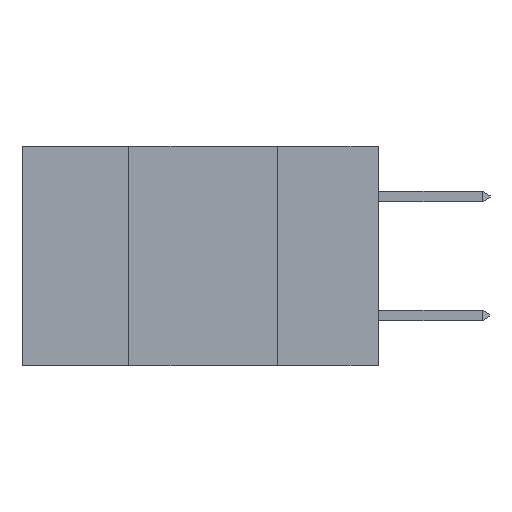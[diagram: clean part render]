
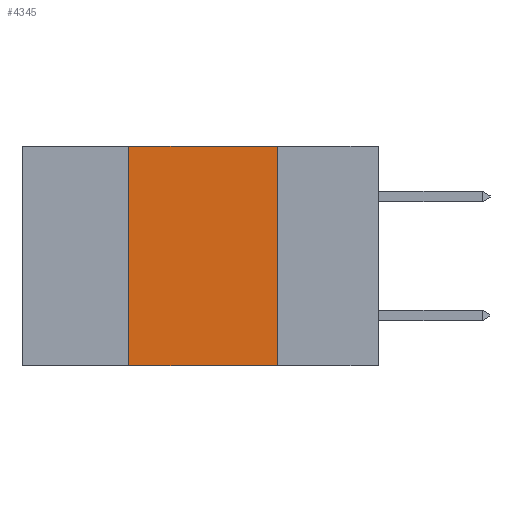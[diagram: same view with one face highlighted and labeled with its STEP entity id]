
A CAD part, left-side view. The second image highlights one B-rep face of the part: STEP entity #4345.
In plain terms, the highlighted planar face has unit normal (-1, 0, 0).
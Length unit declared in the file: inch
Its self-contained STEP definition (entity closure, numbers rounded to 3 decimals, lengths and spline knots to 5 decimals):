
#388 = LINE ( 'NONE', #13098, #13174 ) ;
#1026 = CARTESIAN_POINT ( 'NONE',  ( 0., 0.42, -0.37 ) ) ;
#1184 = VERTEX_POINT ( 'NONE', #21599 ) ;
#2242 = DIRECTION ( 'NONE',  ( 0., -1., 0. ) ) ;
#2478 = LINE ( 'NONE', #9098, #7949 ) ;
#3179 = FACE_OUTER_BOUND ( 'NONE', #18530, .T. ) ;
#3325 = ORIENTED_EDGE ( 'NONE', *, *, #21270, .T. ) ;
#3653 = DIRECTION ( 'NONE',  ( 0., -1., 0. ) ) ;
#3679 = CARTESIAN_POINT ( 'NONE',  ( 0., 0.17, 0. ) ) ;
#4157 = DIRECTION ( 'NONE',  ( 0., 0., -1. ) ) ;
#4345 = ADVANCED_FACE ( 'NONE', ( #3179 ), #14023, .F. ) ;
#6291 = VECTOR ( 'NONE', #14148, 39.37008 ) ;
#6836 = LINE ( 'NONE', #12364, #6291 ) ;
#7418 = VECTOR ( 'NONE', #2242, 39.37008 ) ;
#7736 = VERTEX_POINT ( 'NONE', #15699 ) ;
#7949 = VECTOR ( 'NONE', #3653, 39.37008 ) ;
#7960 = LINE ( 'NONE', #11292, #7418 ) ;
#9098 = CARTESIAN_POINT ( 'NONE',  ( 0., 0.6, 0. ) ) ;
#10260 = VERTEX_POINT ( 'NONE', #1026 ) ;
#11292 = CARTESIAN_POINT ( 'NONE',  ( 0., 0.6, -0.37 ) ) ;
#11504 = AXIS2_PLACEMENT_3D ( 'NONE', #13563, #13070, #12817 ) ;
#11874 = EDGE_CURVE ( 'NONE', #12886, #7736, #388, .T. ) ;
#12364 = CARTESIAN_POINT ( 'NONE',  ( 0., 0.42, -0.37 ) ) ;
#12817 = DIRECTION ( 'NONE',  ( 0., 0., -1. ) ) ;
#12886 = VERTEX_POINT ( 'NONE', #3679 ) ;
#13070 = DIRECTION ( 'NONE',  ( 1., 0., 0. ) ) ;
#13098 = CARTESIAN_POINT ( 'NONE',  ( 0., 0.17, -0.37 ) ) ;
#13174 = VECTOR ( 'NONE', #4157, 39.37008 ) ;
#13463 = ORIENTED_EDGE ( 'NONE', *, *, #18896, .F. ) ;
#13563 = CARTESIAN_POINT ( 'NONE',  ( 0., 0.6, 0. ) ) ;
#14023 = PLANE ( 'NONE',  #11504 ) ;
#14148 = DIRECTION ( 'NONE',  ( 0., 0., 1. ) ) ;
#14541 = ORIENTED_EDGE ( 'NONE', *, *, #11874, .F. ) ;
#15699 = CARTESIAN_POINT ( 'NONE',  ( 0., 0.17, -0.37 ) ) ;
#17738 = EDGE_CURVE ( 'NONE', #1184, #12886, #2478, .T. ) ;
#18530 = EDGE_LOOP ( 'NONE', ( #14541, #18639, #13463, #3325 ) ) ;
#18639 = ORIENTED_EDGE ( 'NONE', *, *, #17738, .F. ) ;
#18896 = EDGE_CURVE ( 'NONE', #10260, #1184, #6836, .T. ) ;
#21270 = EDGE_CURVE ( 'NONE', #10260, #7736, #7960, .T. ) ;
#21599 = CARTESIAN_POINT ( 'NONE',  ( 0., 0.42, 0. ) ) ;
